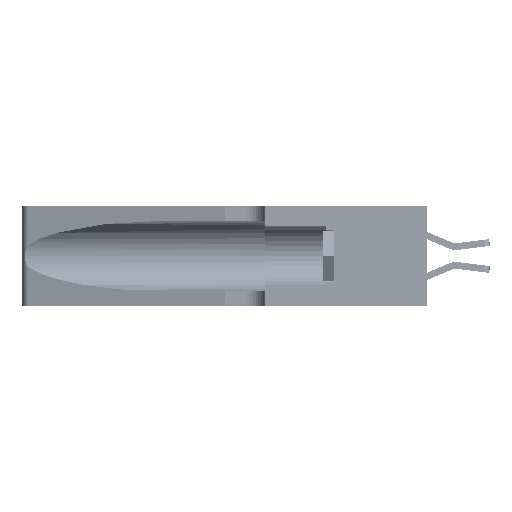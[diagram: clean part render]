
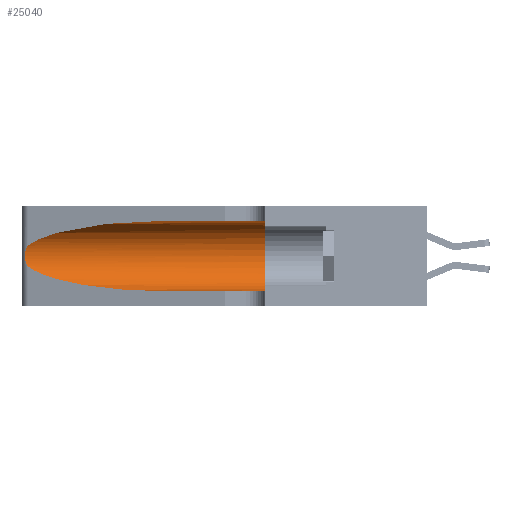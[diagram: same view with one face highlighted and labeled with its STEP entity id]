
A CAD part, left-side view. The second image highlights one B-rep face of the part: STEP entity #25040.
In plain terms, the highlighted cylindrical face has radius 3.308 mm (diameter 6.617 mm), a partial arc.
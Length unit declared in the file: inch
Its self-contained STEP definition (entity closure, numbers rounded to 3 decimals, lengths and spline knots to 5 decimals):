
#705 = CARTESIAN_POINT ( 'NONE',  ( 0.1305, 0.35, 0.05475 ) ) ;
#3112 = EDGE_CURVE ( 'NONE', #34823, #15320, #11208, .T. ) ;
#3356 = CYLINDRICAL_SURFACE ( 'NONE', #8181, 0.13025 ) ;
#4187 = CIRCLE ( 'NONE', #35471, 0.13025 ) ;
#4489 = CARTESIAN_POINT ( 'NONE',  ( 0.2373, 1.15595, 0.08982 ) ) ;
#4536 = VERTEX_POINT ( 'NONE', #17496 ) ;
#4976 = EDGE_CURVE ( 'NONE', #34823, #31782, #27429, .T. ) ;
#5019 = ORIENTED_EDGE ( 'NONE', *, *, #45040, .T. ) ;
#5876 = CARTESIAN_POINT ( 'NONE',  ( 0.25555, 1.22994, 0.2215 ) ) ;
#6719 = CARTESIAN_POINT ( 'NONE',  ( 0.1305, 0.35, 0.185 ) ) ;
#7766 = B_SPLINE_CURVE_WITH_KNOTS ( 'NONE', 3,
 ( #16713, #5876, #20265, #13344, #13642, #41740, #20120, #44988, #20556, #41881, #38016, #41584, #34746, #10062 ),
 .UNSPECIFIED., .F., .F.,
 ( 4, 2, 2, 2, 2, 2, 4 ),
 ( 0., 0.00027, 0.00053, 0.00107, 0.0016, 0.00187, 0.00214 ),
 .UNSPECIFIED. ) ;
#7884 = CARTESIAN_POINT ( 'NONE',  ( 0.1305, 0.72297, 0.05475 ) ) ;
#8181 = AXIS2_PLACEMENT_3D ( 'NONE', #34587, #38172, #41730 ) ;
#8908 = VECTOR ( 'NONE', #42788, 39.37008 ) ;
#9260 = CARTESIAN_POINT ( 'NONE',  ( 0.1305, 0.35, 0.31525 ) ) ;
#10062 = CARTESIAN_POINT ( 'NONE',  ( 0.25487, 1.22718, 0.14631 ) ) ;
#10302 = DIRECTION ( 'NONE',  ( 0., 0., 1. ) ) ;
#11086 = CARTESIAN_POINT ( 'NONE',  ( 0.2373, 1.15595, 0.28018 ) ) ;
#11208 =( BOUNDED_CURVE ( )  B_SPLINE_CURVE ( 3, ( #38574, #27745, #11086, #37280 ),
 .UNSPECIFIED., .F., .F. ) 
 B_SPLINE_CURVE_WITH_KNOTS ( ( 4, 4 ),
 ( 1.5708, 2.84003 ),
 .UNSPECIFIED. ) 
 CURVE ( )  GEOMETRIC_REPRESENTATION_ITEM ( )  RATIONAL_B_SPLINE_CURVE ( ( 1., 0.87, 0.87, 1. ) ) 
 REPRESENTATION_ITEM ( '' )  );
#12958 = CARTESIAN_POINT ( 'NONE',  ( 0.25487, 1.22718, 0.22369 ) ) ;
#13344 = CARTESIAN_POINT ( 'NONE',  ( 0.25787, 1.23484, 0.2124 ) ) ;
#13642 = CARTESIAN_POINT ( 'NONE',  ( 0.25854, 1.2359, 0.20912 ) ) ;
#15320 = VERTEX_POINT ( 'NONE', #12958 ) ;
#16713 = CARTESIAN_POINT ( 'NONE',  ( 0.25487, 1.22718, 0.22369 ) ) ;
#17496 = CARTESIAN_POINT ( 'NONE',  ( 0.1305, 0.72297, 0.05475 ) ) ;
#17797 = EDGE_CURVE ( 'NONE', #15320, #37707, #7766, .T. ) ;
#17908 = CARTESIAN_POINT ( 'NONE',  ( 0.1305, 1.61858, 0.05475 ) ) ;
#18117 = VERTEX_POINT ( 'NONE', #705 ) ;
#19111 =( BOUNDED_CURVE ( )  B_SPLINE_CURVE ( 3, ( #32741, #4489, #25616, #7884 ),
 .UNSPECIFIED., .F., .F. ) 
 B_SPLINE_CURVE_WITH_KNOTS ( ( 4, 4 ),
 ( 3.44316, 4.71239 ),
 .UNSPECIFIED. ) 
 CURVE ( )  GEOMETRIC_REPRESENTATION_ITEM ( )  RATIONAL_B_SPLINE_CURVE ( ( 1., 0.87, 0.87, 1. ) ) 
 REPRESENTATION_ITEM ( '' )  );
#20120 = CARTESIAN_POINT ( 'NONE',  ( 0.26075, 1.23896, 0.19203 ) ) ;
#20265 = CARTESIAN_POINT ( 'NONE',  ( 0.25639, 1.23184, 0.21858 ) ) ;
#20556 = CARTESIAN_POINT ( 'NONE',  ( 0.26017, 1.23833, 0.17102 ) ) ;
#20589 = ORIENTED_EDGE ( 'NONE', *, *, #40519, .T. ) ;
#21012 = ORIENTED_EDGE ( 'NONE', *, *, #37239, .F. ) ;
#24507 = DIRECTION ( 'NONE',  ( 0., -1., 0. ) ) ;
#25040 = ADVANCED_FACE ( 'NONE', ( #39878 ), #3356, .F. ) ;
#25616 = CARTESIAN_POINT ( 'NONE',  ( 0.18966, 0.96281, 0.05475 ) ) ;
#26047 = LINE ( 'NONE', #17908, #8908 ) ;
#27429 = LINE ( 'NONE', #35483, #33502 ) ;
#27671 = CARTESIAN_POINT ( 'NONE',  ( 0.25487, 1.22718, 0.14631 ) ) ;
#27745 = CARTESIAN_POINT ( 'NONE',  ( 0.18966, 0.96281, 0.31525 ) ) ;
#31445 = DIRECTION ( 'NONE',  ( 0., 1., 0. ) ) ;
#31782 = VERTEX_POINT ( 'NONE', #9260 ) ;
#32741 = CARTESIAN_POINT ( 'NONE',  ( 0.25487, 1.22718, 0.14631 ) ) ;
#33502 = VECTOR ( 'NONE', #24507, 39.37008 ) ;
#33873 = EDGE_LOOP ( 'NONE', ( #44007, #44630, #5019, #20589, #21012, #36358 ) ) ;
#34587 = CARTESIAN_POINT ( 'NONE',  ( 0.1305, 1.61858, 0.185 ) ) ;
#34746 = CARTESIAN_POINT ( 'NONE',  ( 0.25555, 1.22993, 0.14849 ) ) ;
#34823 = VERTEX_POINT ( 'NONE', #37717 ) ;
#35471 = AXIS2_PLACEMENT_3D ( 'NONE', #6719, #31445, #10302 ) ;
#35483 = CARTESIAN_POINT ( 'NONE',  ( 0.1305, 1.61858, 0.31525 ) ) ;
#36358 = ORIENTED_EDGE ( 'NONE', *, *, #4976, .F. ) ;
#37239 = EDGE_CURVE ( 'NONE', #31782, #18117, #4187, .T. ) ;
#37280 = CARTESIAN_POINT ( 'NONE',  ( 0.25487, 1.22718, 0.22369 ) ) ;
#37707 = VERTEX_POINT ( 'NONE', #27671 ) ;
#37717 = CARTESIAN_POINT ( 'NONE',  ( 0.1305, 0.72297, 0.31525 ) ) ;
#38016 = CARTESIAN_POINT ( 'NONE',  ( 0.25789, 1.23486, 0.15765 ) ) ;
#38172 = DIRECTION ( 'NONE',  ( 0., -1., 0. ) ) ;
#38574 = CARTESIAN_POINT ( 'NONE',  ( 0.1305, 0.72297, 0.31525 ) ) ;
#39878 = FACE_OUTER_BOUND ( 'NONE', #33873, .T. ) ;
#40519 = EDGE_CURVE ( 'NONE', #4536, #18117, #26047, .T. ) ;
#41584 = CARTESIAN_POINT ( 'NONE',  ( 0.25639, 1.23186, 0.15144 ) ) ;
#41730 = DIRECTION ( 'NONE',  ( 0., 0., -1. ) ) ;
#41740 = CARTESIAN_POINT ( 'NONE',  ( 0.26018, 1.23835, 0.19895 ) ) ;
#41881 = CARTESIAN_POINT ( 'NONE',  ( 0.25856, 1.23593, 0.16098 ) ) ;
#42788 = DIRECTION ( 'NONE',  ( 0., -1., 0. ) ) ;
#44007 = ORIENTED_EDGE ( 'NONE', *, *, #3112, .T. ) ;
#44630 = ORIENTED_EDGE ( 'NONE', *, *, #17797, .T. ) ;
#44988 = CARTESIAN_POINT ( 'NONE',  ( 0.26075, 1.23896, 0.178 ) ) ;
#45040 = EDGE_CURVE ( 'NONE', #37707, #4536, #19111, .T. ) ;
